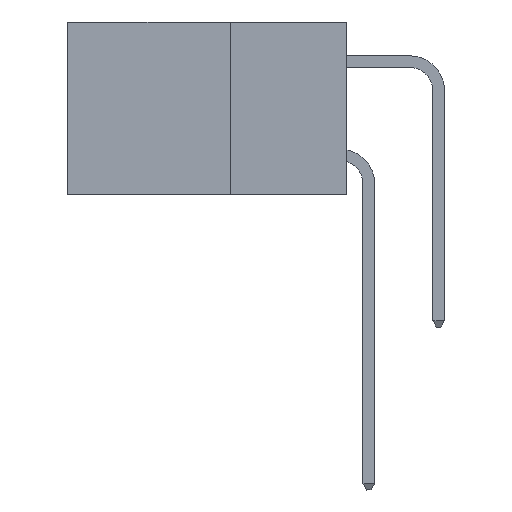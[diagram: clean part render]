
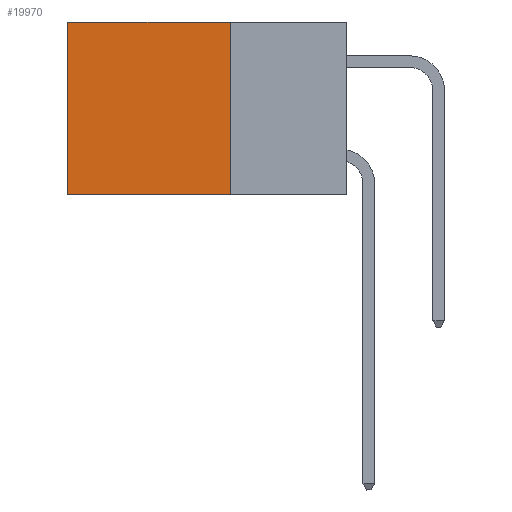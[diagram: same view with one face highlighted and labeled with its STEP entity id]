
A CAD part, left-side view. The second image highlights one B-rep face of the part: STEP entity #19970.
In plain terms, the highlighted planar face has unit normal (-1, 0, 0).
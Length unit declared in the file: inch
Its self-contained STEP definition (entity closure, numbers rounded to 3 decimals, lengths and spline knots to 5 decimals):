
#241 = VERTEX_POINT ( 'NONE', #17271 ) ;
#1461 = VECTOR ( 'NONE', #7124, 39.37008 ) ;
#1674 = CARTESIAN_POINT ( 'NONE',  ( 0.2875, 0.25, -0.37 ) ) ;
#1772 = CARTESIAN_POINT ( 'NONE',  ( 0.2875, 0.25, -0.37 ) ) ;
#1966 = LINE ( 'NONE', #18337, #7109 ) ;
#2269 = ORIENTED_EDGE ( 'NONE', *, *, #23454, .F. ) ;
#2489 = EDGE_CURVE ( 'NONE', #17130, #241, #1966, .T. ) ;
#3688 = VERTEX_POINT ( 'NONE', #1674 ) ;
#3863 = AXIS2_PLACEMENT_3D ( 'NONE', #10809, #24137, #12715 ) ;
#4137 = DIRECTION ( 'NONE',  ( 0., 0., -1. ) ) ;
#6375 = EDGE_LOOP ( 'NONE', ( #12819, #15071, #2269, #24744 ) ) ;
#7095 = VECTOR ( 'NONE', #4137, 39.37008 ) ;
#7109 = VECTOR ( 'NONE', #21301, 39.37008 ) ;
#7124 = DIRECTION ( 'NONE',  ( 0., 1., 0. ) ) ;
#7613 = DIRECTION ( 'NONE',  ( 0., 1., 0. ) ) ;
#8048 = CARTESIAN_POINT ( 'NONE',  ( 0.2875, 0.25, 0. ) ) ;
#8459 = EDGE_CURVE ( 'NONE', #3688, #241, #18767, .T. ) ;
#10734 = PLANE ( 'NONE',  #3863 ) ;
#10809 = CARTESIAN_POINT ( 'NONE',  ( 0.2875, 0.25, 0. ) ) ;
#12715 = DIRECTION ( 'NONE',  ( 0., 0., -1. ) ) ;
#12819 = ORIENTED_EDGE ( 'NONE', *, *, #2489, .T. ) ;
#15071 = ORIENTED_EDGE ( 'NONE', *, *, #8459, .F. ) ;
#16239 = CARTESIAN_POINT ( 'NONE',  ( 0.2875, 0.6, 0. ) ) ;
#16252 = LINE ( 'NONE', #18717, #1461 ) ;
#17130 = VERTEX_POINT ( 'NONE', #16239 ) ;
#17271 = CARTESIAN_POINT ( 'NONE',  ( 0.2875, 0.6, -0.37 ) ) ;
#17322 = LINE ( 'NONE', #8048, #7095 ) ;
#18177 = VECTOR ( 'NONE', #7613, 39.37008 ) ;
#18337 = CARTESIAN_POINT ( 'NONE',  ( 0.2875, 0.6, 0. ) ) ;
#18717 = CARTESIAN_POINT ( 'NONE',  ( 0.2875, 0.25, 0. ) ) ;
#18767 = LINE ( 'NONE', #1772, #18177 ) ;
#19584 = FACE_OUTER_BOUND ( 'NONE', #6375, .T. ) ;
#19970 = ADVANCED_FACE ( 'NONE', ( #19584 ), #10734, .F. ) ;
#20061 = VERTEX_POINT ( 'NONE', #24457 ) ;
#20780 = EDGE_CURVE ( 'NONE', #20061, #17130, #16252, .T. ) ;
#21301 = DIRECTION ( 'NONE',  ( 0., 0., -1. ) ) ;
#23454 = EDGE_CURVE ( 'NONE', #20061, #3688, #17322, .T. ) ;
#24137 = DIRECTION ( 'NONE',  ( 1., 0., 0. ) ) ;
#24457 = CARTESIAN_POINT ( 'NONE',  ( 0.2875, 0.25, 0. ) ) ;
#24744 = ORIENTED_EDGE ( 'NONE', *, *, #20780, .T. ) ;
